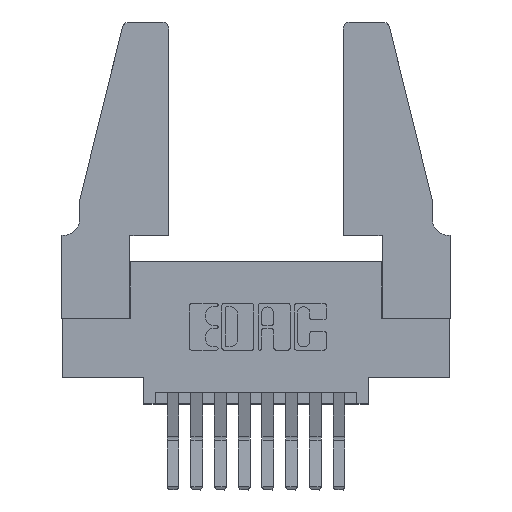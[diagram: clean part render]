
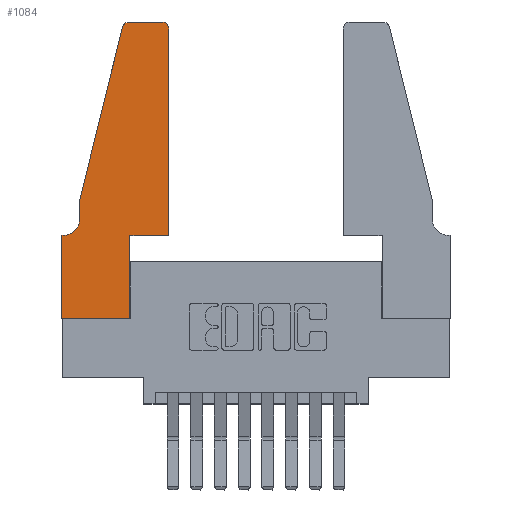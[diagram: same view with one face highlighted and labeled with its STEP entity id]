
A CAD part, top view. The second image highlights one B-rep face of the part: STEP entity #1084.
In plain terms, the highlighted planar face has unit normal (0, 0, 1).
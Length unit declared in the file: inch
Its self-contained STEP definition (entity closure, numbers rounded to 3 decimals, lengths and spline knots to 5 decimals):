
#91 = ORIENTED_EDGE ( 'NONE', *, *, #11975, .T. ) ;
#119 = VECTOR ( 'NONE', #2875, 39.37008 ) ;
#163 = CIRCLE ( 'NONE', #9655, 0.03 ) ;
#179 = CARTESIAN_POINT ( 'NONE',  ( 0.2865, 0.35, 0.37 ) ) ;
#282 = EDGE_LOOP ( 'NONE', ( #6632, #5845, #91, #12521, #2230, #12483, #6134, #6744, #2986, #9549, #3741, #3338 ) ) ;
#510 = VERTEX_POINT ( 'NONE', #1964 ) ;
#804 = VECTOR ( 'NONE', #4499, 39.37008 ) ;
#915 = VERTEX_POINT ( 'NONE', #10984 ) ;
#1084 = ADVANCED_FACE ( 'NONE', ( #11661 ), #2568, .T. ) ;
#1138 = VERTEX_POINT ( 'NONE', #5060 ) ;
#1475 = DIRECTION ( 'NONE',  ( 1., 0., 0. ) ) ;
#1517 = CARTESIAN_POINT ( 'NONE',  ( 0., 0., 0.37 ) ) ;
#1533 = EDGE_CURVE ( 'NONE', #4751, #510, #9309, .T. ) ;
#1728 = CARTESIAN_POINT ( 'NONE',  ( 0.2605, 1.25, 0.37 ) ) ;
#1964 = CARTESIAN_POINT ( 'NONE',  ( 0.4505, 1.22, 0.37 ) ) ;
#2170 = VERTEX_POINT ( 'NONE', #2264 ) ;
#2177 = EDGE_CURVE ( 'NONE', #2318, #6342, #4789, .T. ) ;
#2230 = ORIENTED_EDGE ( 'NONE', *, *, #2177, .T. ) ;
#2264 = CARTESIAN_POINT ( 'NONE',  ( 0., 0., 0.37 ) ) ;
#2318 = VERTEX_POINT ( 'NONE', #11644 ) ;
#2452 = CARTESIAN_POINT ( 'NONE',  ( 0.2865, 0.35, 0.37 ) ) ;
#2568 = PLANE ( 'NONE',  #8226 ) ;
#2650 = CARTESIAN_POINT ( 'NONE',  ( 0.4205, 1.22, 0.37 ) ) ;
#2875 = DIRECTION ( 'NONE',  ( -0.239, -0.971, 0. ) ) ;
#2986 = ORIENTED_EDGE ( 'NONE', *, *, #12349, .T. ) ;
#3338 = ORIENTED_EDGE ( 'NONE', *, *, #10620, .T. ) ;
#3422 = DIRECTION ( 'NONE',  ( 0., -1., 0. ) ) ;
#3616 = VERTEX_POINT ( 'NONE', #9697 ) ;
#3683 = DIRECTION ( 'NONE',  ( 1., 0., 0. ) ) ;
#3741 = ORIENTED_EDGE ( 'NONE', *, *, #1533, .T. ) ;
#4324 = VECTOR ( 'NONE', #7671, 39.37008 ) ;
#4411 = CARTESIAN_POINT ( 'NONE',  ( 0.4505, 0.35, 0.37 ) ) ;
#4499 = DIRECTION ( 'NONE',  ( 0., 1., 0. ) ) ;
#4648 = VERTEX_POINT ( 'NONE', #8444 ) ;
#4751 = VERTEX_POINT ( 'NONE', #6583 ) ;
#4789 = CIRCLE ( 'NONE', #10829, 0.07 ) ;
#4800 = DIRECTION ( 'NONE',  ( -1., 0., 0. ) ) ;
#4858 = DIRECTION ( 'NONE',  ( -1., 0., 0. ) ) ;
#5060 = CARTESIAN_POINT ( 'NONE',  ( 0.25487, 1.22718, 0.37 ) ) ;
#5124 = EDGE_CURVE ( 'NONE', #6342, #13123, #13224, .T. ) ;
#5200 = LINE ( 'NONE', #7479, #12998 ) ;
#5220 = LINE ( 'NONE', #7633, #13013 ) ;
#5356 = DIRECTION ( 'NONE',  ( 0., 0., -1. ) ) ;
#5418 = DIRECTION ( 'NONE',  ( 1., 0., 0. ) ) ;
#5646 = LINE ( 'NONE', #5880, #119 ) ;
#5807 = CARTESIAN_POINT ( 'NONE',  ( 0.284, 1.22, 0.37 ) ) ;
#5845 = ORIENTED_EDGE ( 'NONE', *, *, #6984, .T. ) ;
#5880 = CARTESIAN_POINT ( 'NONE',  ( 0.0755, 0.5, 0.37 ) ) ;
#5976 = VECTOR ( 'NONE', #4800, 39.37008 ) ;
#6134 = ORIENTED_EDGE ( 'NONE', *, *, #6873, .T. ) ;
#6191 = DIRECTION ( 'NONE',  ( 0., 1., 0. ) ) ;
#6286 = CARTESIAN_POINT ( 'NONE',  ( 0.4205, 1.25, 0.37 ) ) ;
#6342 = VERTEX_POINT ( 'NONE', #11654 ) ;
#6583 = CARTESIAN_POINT ( 'NONE',  ( 0.4505, 0.35, 0.37 ) ) ;
#6631 = DIRECTION ( 'NONE',  ( 0., 0., 1. ) ) ;
#6632 = ORIENTED_EDGE ( 'NONE', *, *, #11942, .T. ) ;
#6744 = ORIENTED_EDGE ( 'NONE', *, *, #9286, .T. ) ;
#6866 = DIRECTION ( 'NONE',  ( 1., 0., 0. ) ) ;
#6873 = EDGE_CURVE ( 'NONE', #13123, #2170, #9770, .T. ) ;
#6984 = EDGE_CURVE ( 'NONE', #915, #1138, #10860, .T. ) ;
#7479 = CARTESIAN_POINT ( 'NONE',  ( 0.0755, 0.5, 0.37 ) ) ;
#7633 = CARTESIAN_POINT ( 'NONE',  ( 0.4505, 0.35, 0.37 ) ) ;
#7671 = DIRECTION ( 'NONE',  ( 0., -1., 0. ) ) ;
#7993 = CARTESIAN_POINT ( 'NONE',  ( 0.0755, 0.35, 0.37 ) ) ;
#8085 = EDGE_CURVE ( 'NONE', #8613, #4751, #5220, .T. ) ;
#8226 = AXIS2_PLACEMENT_3D ( 'NONE', #9009, #6631, #9305 ) ;
#8444 = CARTESIAN_POINT ( 'NONE',  ( 0.0755, 0.5, 0.37 ) ) ;
#8613 = VERTEX_POINT ( 'NONE', #179 ) ;
#8731 = LINE ( 'NONE', #1728, #5976 ) ;
#9009 = CARTESIAN_POINT ( 'NONE',  ( 0., 0.35, 0.37 ) ) ;
#9286 = EDGE_CURVE ( 'NONE', #2170, #3616, #9726, .T. ) ;
#9305 = DIRECTION ( 'NONE',  ( 1., 0., 0. ) ) ;
#9309 = LINE ( 'NONE', #4411, #9929 ) ;
#9549 = ORIENTED_EDGE ( 'NONE', *, *, #8085, .T. ) ;
#9655 = AXIS2_PLACEMENT_3D ( 'NONE', #2650, #9799, #3683 ) ;
#9697 = CARTESIAN_POINT ( 'NONE',  ( 0.2865, 0., 0.37 ) ) ;
#9726 = LINE ( 'NONE', #12537, #12063 ) ;
#9770 = LINE ( 'NONE', #1517, #4324 ) ;
#9799 = DIRECTION ( 'NONE',  ( 0., 0., 1. ) ) ;
#9929 = VECTOR ( 'NONE', #6191, 39.37008 ) ;
#10281 = VECTOR ( 'NONE', #4858, 39.37008 ) ;
#10467 = EDGE_CURVE ( 'NONE', #4648, #2318, #5200, .T. ) ;
#10620 = EDGE_CURVE ( 'NONE', #510, #10959, #163, .T. ) ;
#10829 = AXIS2_PLACEMENT_3D ( 'NONE', #11471, #5356, #12467 ) ;
#10860 = CIRCLE ( 'NONE', #10871, 0.03 ) ;
#10871 = AXIS2_PLACEMENT_3D ( 'NONE', #5807, #12902, #6866 ) ;
#10959 = VERTEX_POINT ( 'NONE', #6286 ) ;
#10984 = CARTESIAN_POINT ( 'NONE',  ( 0.284, 1.25, 0.37 ) ) ;
#11471 = CARTESIAN_POINT ( 'NONE',  ( 0.0055, 0.42, 0.37 ) ) ;
#11644 = CARTESIAN_POINT ( 'NONE',  ( 0.0755, 0.42, 0.37 ) ) ;
#11654 = CARTESIAN_POINT ( 'NONE',  ( 0.0055, 0.35, 0.37 ) ) ;
#11661 = FACE_OUTER_BOUND ( 'NONE', #282, .T. ) ;
#11942 = EDGE_CURVE ( 'NONE', #10959, #915, #8731, .T. ) ;
#11975 = EDGE_CURVE ( 'NONE', #1138, #4648, #5646, .T. ) ;
#12007 = LINE ( 'NONE', #2452, #804 ) ;
#12063 = VECTOR ( 'NONE', #5418, 39.37008 ) ;
#12349 = EDGE_CURVE ( 'NONE', #3616, #8613, #12007, .T. ) ;
#12467 = DIRECTION ( 'NONE',  ( -1., 0., 0. ) ) ;
#12483 = ORIENTED_EDGE ( 'NONE', *, *, #5124, .T. ) ;
#12521 = ORIENTED_EDGE ( 'NONE', *, *, #10467, .T. ) ;
#12537 = CARTESIAN_POINT ( 'NONE',  ( 0., 0., 0.37 ) ) ;
#12772 = CARTESIAN_POINT ( 'NONE',  ( 0., 0.35, 0.37 ) ) ;
#12902 = DIRECTION ( 'NONE',  ( 0., 0., 1. ) ) ;
#12998 = VECTOR ( 'NONE', #3422, 39.37008 ) ;
#13013 = VECTOR ( 'NONE', #1475, 39.37008 ) ;
#13123 = VERTEX_POINT ( 'NONE', #12772 ) ;
#13224 = LINE ( 'NONE', #7993, #10281 ) ;
